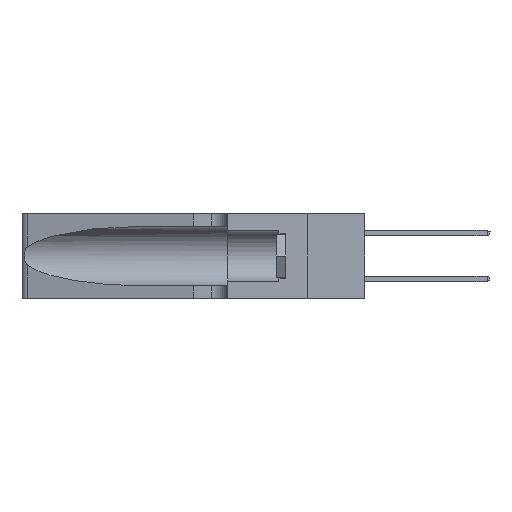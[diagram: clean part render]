
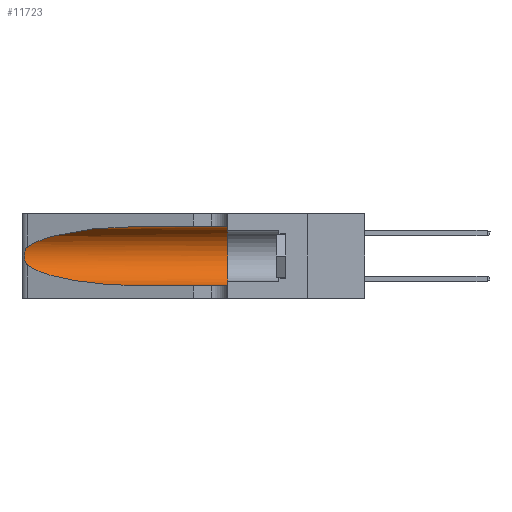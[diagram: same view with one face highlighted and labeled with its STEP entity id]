
A CAD part, left-side view. The second image highlights one B-rep face of the part: STEP entity #11723.
In plain terms, the highlighted cylindrical face has radius 3.308 mm (diameter 6.617 mm), a partial arc.
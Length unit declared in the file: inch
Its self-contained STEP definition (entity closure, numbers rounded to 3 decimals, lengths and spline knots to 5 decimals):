
#120 = CARTESIAN_POINT ( 'NONE',  ( 0.25789, 1.23486, 0.15765 ) ) ;
#246 = CARTESIAN_POINT ( 'NONE',  ( 0.1305, 1.61858, 0.05475 ) ) ;
#311 = VERTEX_POINT ( 'NONE', #8475 ) ;
#675 = CARTESIAN_POINT ( 'NONE',  ( 0.1305, 0.72297, 0.31525 ) ) ;
#711 = AXIS2_PLACEMENT_3D ( 'NONE', #24260, #7655, #27001 ) ;
#1126 = FACE_OUTER_BOUND ( 'NONE', #23234, .T. ) ;
#2938 = CARTESIAN_POINT ( 'NONE',  ( 0.25555, 1.22993, 0.14849 ) ) ;
#3521 = CARTESIAN_POINT ( 'NONE',  ( 0.2373, 1.15595, 0.28018 ) ) ;
#3643 = DIRECTION ( 'NONE',  ( 0., -1., 0. ) ) ;
#5190 = VECTOR ( 'NONE', #3643, 39.37008 ) ;
#7655 = DIRECTION ( 'NONE',  ( 0., 1., 0. ) ) ;
#8287 = VERTEX_POINT ( 'NONE', #13247 ) ;
#8312 = CARTESIAN_POINT ( 'NONE',  ( 0.25555, 1.22994, 0.2215 ) ) ;
#8438 = CARTESIAN_POINT ( 'NONE',  ( 0.25787, 1.23484, 0.2124 ) ) ;
#8475 = CARTESIAN_POINT ( 'NONE',  ( 0.1305, 0.72297, 0.05475 ) ) ;
#8632 = VERTEX_POINT ( 'NONE', #675 ) ;
#8895 = ORIENTED_EDGE ( 'NONE', *, *, #29153, .T. ) ;
#9921 =( BOUNDED_CURVE ( )  B_SPLINE_CURVE ( 3, ( #24237, #21452, #13235, #32506 ),
 .UNSPECIFIED., .F., .T. ) 
 B_SPLINE_CURVE_WITH_KNOTS ( ( 4, 4 ),
 ( 3.44316, 4.71239 ),
 .UNSPECIFIED. ) 
 CURVE ( )  GEOMETRIC_REPRESENTATION_ITEM ( )  RATIONAL_B_SPLINE_CURVE ( ( 1., 0.87, 0.87, 1. ) ) 
 REPRESENTATION_ITEM ( '' )  );
#10035 = DIRECTION ( 'NONE',  ( 0., -1., 0. ) ) ;
#10068 = LINE ( 'NONE', #246, #22176 ) ;
#10080 = EDGE_CURVE ( 'NONE', #8632, #18463, #20845, .T. ) ;
#11248 = CARTESIAN_POINT ( 'NONE',  ( 0.26018, 1.23835, 0.19895 ) ) ;
#11723 = ADVANCED_FACE ( 'NONE', ( #1126 ), #21543, .F. ) ;
#12597 = ORIENTED_EDGE ( 'NONE', *, *, #15600, .T. ) ;
#13235 = CARTESIAN_POINT ( 'NONE',  ( 0.18966, 0.96281, 0.05475 ) ) ;
#13247 = CARTESIAN_POINT ( 'NONE',  ( 0.25487, 1.22718, 0.22369 ) ) ;
#13444 = CARTESIAN_POINT ( 'NONE',  ( 0.25487, 1.22718, 0.14631 ) ) ;
#14004 = CARTESIAN_POINT ( 'NONE',  ( 0.26075, 1.23896, 0.178 ) ) ;
#14581 = CARTESIAN_POINT ( 'NONE',  ( 0.18966, 0.96281, 0.31525 ) ) ;
#15557 = EDGE_CURVE ( 'NONE', #8287, #31514, #22775, .T. ) ;
#15600 = EDGE_CURVE ( 'NONE', #311, #25926, #10068, .T. ) ;
#16807 = CARTESIAN_POINT ( 'NONE',  ( 0.25856, 1.23593, 0.16098 ) ) ;
#18463 = VERTEX_POINT ( 'NONE', #30162 ) ;
#19136 = ORIENTED_EDGE ( 'NONE', *, *, #10080, .F. ) ;
#19275 = ORIENTED_EDGE ( 'NONE', *, *, #19737, .T. ) ;
#19447 = CARTESIAN_POINT ( 'NONE',  ( 0.25487, 1.22718, 0.22369 ) ) ;
#19567 = CARTESIAN_POINT ( 'NONE',  ( 0.25639, 1.23186, 0.15144 ) ) ;
#19737 = EDGE_CURVE ( 'NONE', #31514, #311, #9921, .T. ) ;
#20118 =( BOUNDED_CURVE ( )  B_SPLINE_CURVE ( 3, ( #31091, #14581, #3521, #22926 ),
 .UNSPECIFIED., .F., .T. ) 
 B_SPLINE_CURVE_WITH_KNOTS ( ( 4, 4 ),
 ( 1.5708, 2.84003 ),
 .UNSPECIFIED. ) 
 CURVE ( )  GEOMETRIC_REPRESENTATION_ITEM ( )  RATIONAL_B_SPLINE_CURVE ( ( 1., 0.87, 0.87, 1. ) ) 
 REPRESENTATION_ITEM ( '' )  );
#20845 = LINE ( 'NONE', #28540, #5190 ) ;
#21048 = DIRECTION ( 'NONE',  ( 0., 0., -1. ) ) ;
#21452 = CARTESIAN_POINT ( 'NONE',  ( 0.2373, 1.15595, 0.08982 ) ) ;
#21543 = CYLINDRICAL_SURFACE ( 'NONE', #26881, 0.13025 ) ;
#22129 = CARTESIAN_POINT ( 'NONE',  ( 0.1305, 0.35, 0.05475 ) ) ;
#22176 = VECTOR ( 'NONE', #33386, 39.37008 ) ;
#22358 = CARTESIAN_POINT ( 'NONE',  ( 0.25487, 1.22718, 0.14631 ) ) ;
#22775 = B_SPLINE_CURVE_WITH_KNOTS ( 'NONE', 3,
 ( #19447, #8312, #25019, #8438, #27759, #11248, #30512, #14004, #33272, #16807, #120, #19567, #2938, #22358 ),
 .UNSPECIFIED., .F., .F.,
 ( 4, 2, 2, 2, 2, 2, 4 ),
 ( 0., 0.00027, 0.00053, 0.00107, 0.0016, 0.00187, 0.00214 ),
 .UNSPECIFIED. ) ;
#22926 = CARTESIAN_POINT ( 'NONE',  ( 0.25487, 1.22718, 0.22369 ) ) ;
#23234 = EDGE_LOOP ( 'NONE', ( #8895, #33219, #19275, #12597, #26610, #19136 ) ) ;
#23850 = CARTESIAN_POINT ( 'NONE',  ( 0.1305, 1.61858, 0.185 ) ) ;
#24237 = CARTESIAN_POINT ( 'NONE',  ( 0.25487, 1.22718, 0.14631 ) ) ;
#24260 = CARTESIAN_POINT ( 'NONE',  ( 0.1305, 0.35, 0.185 ) ) ;
#25019 = CARTESIAN_POINT ( 'NONE',  ( 0.25639, 1.23184, 0.21858 ) ) ;
#25926 = VERTEX_POINT ( 'NONE', #22129 ) ;
#26610 = ORIENTED_EDGE ( 'NONE', *, *, #33313, .F. ) ;
#26881 = AXIS2_PLACEMENT_3D ( 'NONE', #23850, #10035, #21048 ) ;
#27001 = DIRECTION ( 'NONE',  ( 0., 0., 1. ) ) ;
#27759 = CARTESIAN_POINT ( 'NONE',  ( 0.25854, 1.2359, 0.20912 ) ) ;
#28540 = CARTESIAN_POINT ( 'NONE',  ( 0.1305, 1.61858, 0.31525 ) ) ;
#28918 = CIRCLE ( 'NONE', #711, 0.13025 ) ;
#29153 = EDGE_CURVE ( 'NONE', #8632, #8287, #20118, .T. ) ;
#30162 = CARTESIAN_POINT ( 'NONE',  ( 0.1305, 0.35, 0.31525 ) ) ;
#30512 = CARTESIAN_POINT ( 'NONE',  ( 0.26075, 1.23896, 0.19203 ) ) ;
#31091 = CARTESIAN_POINT ( 'NONE',  ( 0.1305, 0.72297, 0.31525 ) ) ;
#31514 = VERTEX_POINT ( 'NONE', #13444 ) ;
#32506 = CARTESIAN_POINT ( 'NONE',  ( 0.1305, 0.72297, 0.05475 ) ) ;
#33219 = ORIENTED_EDGE ( 'NONE', *, *, #15557, .T. ) ;
#33272 = CARTESIAN_POINT ( 'NONE',  ( 0.26017, 1.23833, 0.17102 ) ) ;
#33313 = EDGE_CURVE ( 'NONE', #18463, #25926, #28918, .T. ) ;
#33386 = DIRECTION ( 'NONE',  ( 0., -1., 0. ) ) ;
